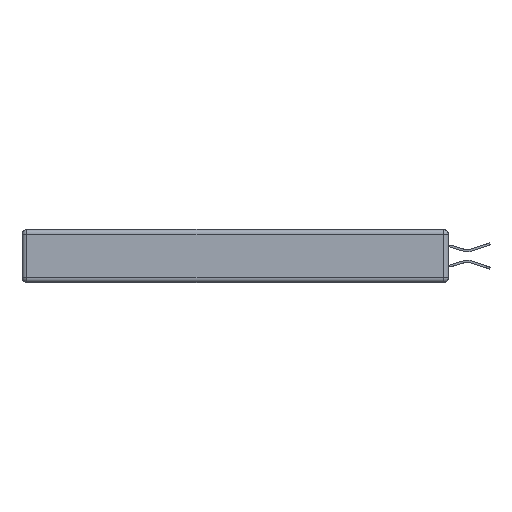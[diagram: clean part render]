
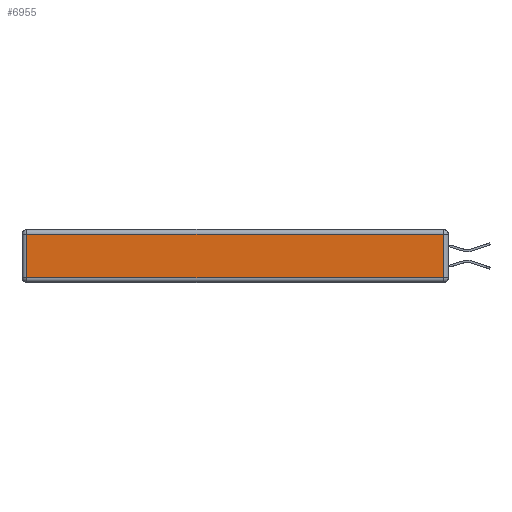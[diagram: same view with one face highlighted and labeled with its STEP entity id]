
A CAD part, left-side view. The second image highlights one B-rep face of the part: STEP entity #6955.
In plain terms, the highlighted planar face has unit normal (-1, 0, 0).
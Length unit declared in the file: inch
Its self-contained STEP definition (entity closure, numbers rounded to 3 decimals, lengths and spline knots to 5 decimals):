
#127 = CARTESIAN_POINT ( 'NONE',  ( 0., 2.72, -0.313 ) ) ;
#386 = CARTESIAN_POINT ( 'NONE',  ( 0., 0.03, -0.343 ) ) ;
#502 = CARTESIAN_POINT ( 'NONE',  ( 0., 0.03, -0.313 ) ) ;
#553 = DIRECTION ( 'NONE',  ( 0., 0., 1. ) ) ;
#864 = DIRECTION ( 'NONE',  ( 0., -1., 0. ) ) ;
#1088 = CARTESIAN_POINT ( 'NONE',  ( 0., 2.75, -0.03 ) ) ;
#3296 = EDGE_CURVE ( 'NONE', #19725, #17582, #21001, .T. ) ;
#4847 = DIRECTION ( 'NONE',  ( 0., 1., 0. ) ) ;
#6955 = ADVANCED_FACE ( 'NONE', ( #15769 ), #23037, .T. ) ;
#7595 = ORIENTED_EDGE ( 'NONE', *, *, #18880, .T. ) ;
#8696 = VERTEX_POINT ( 'NONE', #502 ) ;
#8908 = EDGE_LOOP ( 'NONE', ( #23680, #20741, #7595, #17064 ) ) ;
#10216 = VECTOR ( 'NONE', #4847, 39.37008 ) ;
#14898 = LINE ( 'NONE', #1088, #10216 ) ;
#15769 = FACE_OUTER_BOUND ( 'NONE', #8908, .T. ) ;
#15941 = VECTOR ( 'NONE', #864, 39.37008 ) ;
#16437 = CARTESIAN_POINT ( 'NONE',  ( 0., 2.72, -0.343 ) ) ;
#16605 = VECTOR ( 'NONE', #20464, 39.37008 ) ;
#17064 = ORIENTED_EDGE ( 'NONE', *, *, #3296, .T. ) ;
#17468 = VECTOR ( 'NONE', #553, 39.37008 ) ;
#17582 = VERTEX_POINT ( 'NONE', #127 ) ;
#17593 = CARTESIAN_POINT ( 'NONE',  ( 0., 2.72, -0.03 ) ) ;
#17721 = VERTEX_POINT ( 'NONE', #22936 ) ;
#18880 = EDGE_CURVE ( 'NONE', #17721, #19725, #14898, .T. ) ;
#18988 = AXIS2_PLACEMENT_3D ( 'NONE', #21148, #21312, #23122 ) ;
#19725 = VERTEX_POINT ( 'NONE', #17593 ) ;
#20464 = DIRECTION ( 'NONE',  ( 0., 0., -1. ) ) ;
#20741 = ORIENTED_EDGE ( 'NONE', *, *, #23169, .T. ) ;
#21001 = LINE ( 'NONE', #16437, #16605 ) ;
#21148 = CARTESIAN_POINT ( 'NONE',  ( 0., 0., -0.343 ) ) ;
#21312 = DIRECTION ( 'NONE',  ( -1., 0., 0. ) ) ;
#22459 = EDGE_CURVE ( 'NONE', #17582, #8696, #24985, .T. ) ;
#22770 = LINE ( 'NONE', #386, #17468 ) ;
#22936 = CARTESIAN_POINT ( 'NONE',  ( 0., 0.03, -0.03 ) ) ;
#23037 = PLANE ( 'NONE',  #18988 ) ;
#23122 = DIRECTION ( 'NONE',  ( 0., 0., 1. ) ) ;
#23169 = EDGE_CURVE ( 'NONE', #8696, #17721, #22770, .T. ) ;
#23680 = ORIENTED_EDGE ( 'NONE', *, *, #22459, .T. ) ;
#24985 = LINE ( 'NONE', #25055, #15941 ) ;
#25055 = CARTESIAN_POINT ( 'NONE',  ( 0., 0., -0.313 ) ) ;
